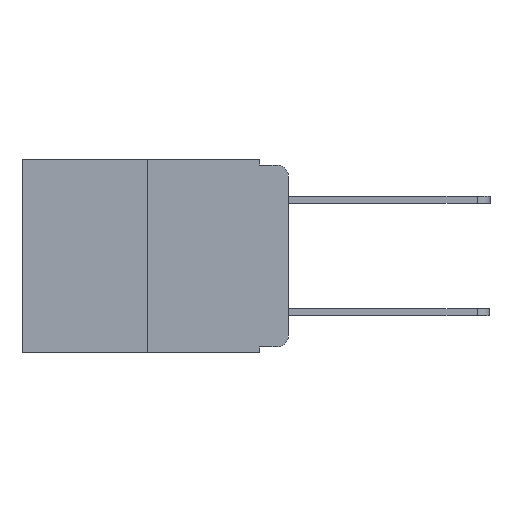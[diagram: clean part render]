
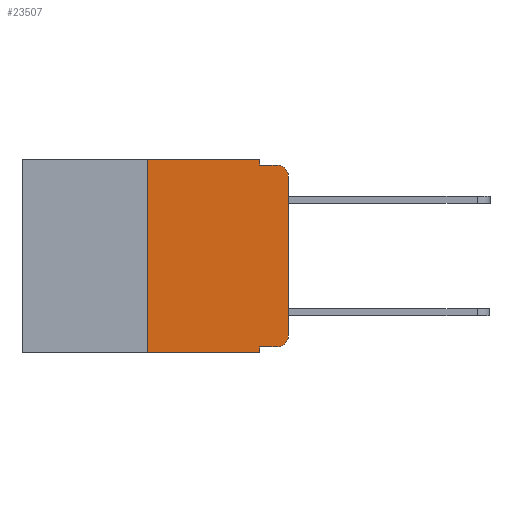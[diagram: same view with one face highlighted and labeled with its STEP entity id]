
A CAD part, left-side view. The second image highlights one B-rep face of the part: STEP entity #23507.
In plain terms, the highlighted planar face has unit normal (-1, 0, 0).
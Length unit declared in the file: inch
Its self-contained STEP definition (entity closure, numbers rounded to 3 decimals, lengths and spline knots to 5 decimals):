
#71 = CARTESIAN_POINT ( 'NONE',  ( 0., 0.02, -0.03 ) ) ;
#109 = EDGE_LOOP ( 'NONE', ( #22096, #17200, #16670, #16168, #15599, #14370, #13208, #13432, #20068, #18311 ) ) ;
#448 = LINE ( 'NONE', #855, #15501 ) ;
#730 = VECTOR ( 'NONE', #10645, 39.37008 ) ;
#855 = CARTESIAN_POINT ( 'NONE',  ( 0., 0.473, -0.343 ) ) ;
#973 = VECTOR ( 'NONE', #9719, 39.37008 ) ;
#1287 = AXIS2_PLACEMENT_3D ( 'NONE', #13037, #18853, #7346 ) ;
#2120 = DIRECTION ( 'NONE',  ( 0., 0., -1. ) ) ;
#2637 = VERTEX_POINT ( 'NONE', #23404 ) ;
#2841 = LINE ( 'NONE', #17798, #15955 ) ;
#2913 = DIRECTION ( 'NONE',  ( 0., -1., 0. ) ) ;
#3238 = VERTEX_POINT ( 'NONE', #15653 ) ;
#4207 = EDGE_CURVE ( 'NONE', #20473, #3238, #8319, .T. ) ;
#4243 = LINE ( 'NONE', #23338, #8882 ) ;
#4558 = EDGE_CURVE ( 'NONE', #3238, #19817, #17620, .T. ) ;
#4857 = DIRECTION ( 'NONE',  ( -1., 0., 0. ) ) ;
#5067 = EDGE_CURVE ( 'NONE', #13266, #14023, #4243, .T. ) ;
#5573 = DIRECTION ( 'NONE',  ( 0., 0., 1. ) ) ;
#5690 = VECTOR ( 'NONE', #19800, 39.37008 ) ;
#5757 = FACE_OUTER_BOUND ( 'NONE', #109, .T. ) ;
#6110 = CARTESIAN_POINT ( 'NONE',  ( 0., 0.25, -0.343 ) ) ;
#6320 = LINE ( 'NONE', #23490, #5690 ) ;
#6620 = DIRECTION ( 'NONE',  ( 0., 0., 1. ) ) ;
#7346 = DIRECTION ( 'NONE',  ( 0., 0., -1. ) ) ;
#7542 = VERTEX_POINT ( 'NONE', #19670 ) ;
#7582 = CARTESIAN_POINT ( 'NONE',  ( 0., 0.25, 0. ) ) ;
#7648 = VECTOR ( 'NONE', #5573, 39.37008 ) ;
#7810 = CARTESIAN_POINT ( 'NONE',  ( 0., 0.051, -0.01 ) ) ;
#8319 = CIRCLE ( 'NONE', #9571, 0.02 ) ;
#8747 = VERTEX_POINT ( 'NONE', #6110 ) ;
#8782 = CARTESIAN_POINT ( 'NONE',  ( 0., 0.473, 0. ) ) ;
#8882 = VECTOR ( 'NONE', #10027, 39.37008 ) ;
#9571 = AXIS2_PLACEMENT_3D ( 'NONE', #16445, #4857, #18386 ) ;
#9719 = DIRECTION ( 'NONE',  ( 0., -1., 0. ) ) ;
#10027 = DIRECTION ( 'NONE',  ( 0., 0., -1. ) ) ;
#10332 = CARTESIAN_POINT ( 'NONE',  ( 0., 0.02, -0.333 ) ) ;
#10645 = DIRECTION ( 'NONE',  ( 0., -1., 0. ) ) ;
#10711 = EDGE_CURVE ( 'NONE', #2637, #20473, #2841, .T. ) ;
#13037 = CARTESIAN_POINT ( 'NONE',  ( 0., 0.473, 0. ) ) ;
#13208 = ORIENTED_EDGE ( 'NONE', *, *, #19982, .T. ) ;
#13266 = VERTEX_POINT ( 'NONE', #21989 ) ;
#13432 = ORIENTED_EDGE ( 'NONE', *, *, #15925, .F. ) ;
#13824 = DIRECTION ( 'NONE',  ( -1., 0., 0. ) ) ;
#14023 = VERTEX_POINT ( 'NONE', #14675 ) ;
#14289 = CARTESIAN_POINT ( 'NONE',  ( 0., 0., 0. ) ) ;
#14370 = ORIENTED_EDGE ( 'NONE', *, *, #22316, .F. ) ;
#14675 = CARTESIAN_POINT ( 'NONE',  ( 0., 0.051, -0.01 ) ) ;
#15419 = AXIS2_PLACEMENT_3D ( 'NONE', #71, #13824, #2120 ) ;
#15449 = EDGE_CURVE ( 'NONE', #14023, #7542, #17212, .T. ) ;
#15501 = VECTOR ( 'NONE', #2913, 39.37008 ) ;
#15599 = ORIENTED_EDGE ( 'NONE', *, *, #20572, .F. ) ;
#15653 = CARTESIAN_POINT ( 'NONE',  ( 0., 0., -0.313 ) ) ;
#15865 = VERTEX_POINT ( 'NONE', #20390 ) ;
#15925 = EDGE_CURVE ( 'NONE', #2637, #15865, #6320, .T. ) ;
#15955 = VECTOR ( 'NONE', #23406, 39.37008 ) ;
#16168 = ORIENTED_EDGE ( 'NONE', *, *, #5067, .F. ) ;
#16374 = LINE ( 'NONE', #8782, #730 ) ;
#16445 = CARTESIAN_POINT ( 'NONE',  ( 0., 0.02, -0.313 ) ) ;
#16670 = ORIENTED_EDGE ( 'NONE', *, *, #15449, .F. ) ;
#17200 = ORIENTED_EDGE ( 'NONE', *, *, #23090, .T. ) ;
#17212 = LINE ( 'NONE', #7810, #973 ) ;
#17620 = LINE ( 'NONE', #14289, #21478 ) ;
#17798 = CARTESIAN_POINT ( 'NONE',  ( 0., 0.051, -0.333 ) ) ;
#17887 = LINE ( 'NONE', #7582, #7648 ) ;
#18311 = ORIENTED_EDGE ( 'NONE', *, *, #4207, .T. ) ;
#18386 = DIRECTION ( 'NONE',  ( 0., 0., -1. ) ) ;
#18853 = DIRECTION ( 'NONE',  ( 1., 0., 0. ) ) ;
#19670 = CARTESIAN_POINT ( 'NONE',  ( 0., 0.02, -0.01 ) ) ;
#19800 = DIRECTION ( 'NONE',  ( 0., 0., -1. ) ) ;
#19817 = VERTEX_POINT ( 'NONE', #23253 ) ;
#19982 = EDGE_CURVE ( 'NONE', #8747, #15865, #448, .T. ) ;
#19989 = CIRCLE ( 'NONE', #15419, 0.02 ) ;
#20068 = ORIENTED_EDGE ( 'NONE', *, *, #10711, .T. ) ;
#20233 = VERTEX_POINT ( 'NONE', #22916 ) ;
#20390 = CARTESIAN_POINT ( 'NONE',  ( 0., 0.051, -0.343 ) ) ;
#20473 = VERTEX_POINT ( 'NONE', #10332 ) ;
#20572 = EDGE_CURVE ( 'NONE', #20233, #13266, #16374, .T. ) ;
#21478 = VECTOR ( 'NONE', #6620, 39.37008 ) ;
#21989 = CARTESIAN_POINT ( 'NONE',  ( 0., 0.051, 0. ) ) ;
#22096 = ORIENTED_EDGE ( 'NONE', *, *, #4558, .T. ) ;
#22316 = EDGE_CURVE ( 'NONE', #8747, #20233, #17887, .T. ) ;
#22589 = PLANE ( 'NONE',  #1287 ) ;
#22916 = CARTESIAN_POINT ( 'NONE',  ( 0., 0.25, 0. ) ) ;
#23090 = EDGE_CURVE ( 'NONE', #19817, #7542, #19989, .T. ) ;
#23253 = CARTESIAN_POINT ( 'NONE',  ( 0., 0., -0.03 ) ) ;
#23338 = CARTESIAN_POINT ( 'NONE',  ( 0., 0.051, 0. ) ) ;
#23404 = CARTESIAN_POINT ( 'NONE',  ( 0., 0.051, -0.333 ) ) ;
#23406 = DIRECTION ( 'NONE',  ( 0., -1., 0. ) ) ;
#23490 = CARTESIAN_POINT ( 'NONE',  ( 0., 0.051, 0. ) ) ;
#23507 = ADVANCED_FACE ( 'NONE', ( #5757 ), #22589, .F. ) ;
